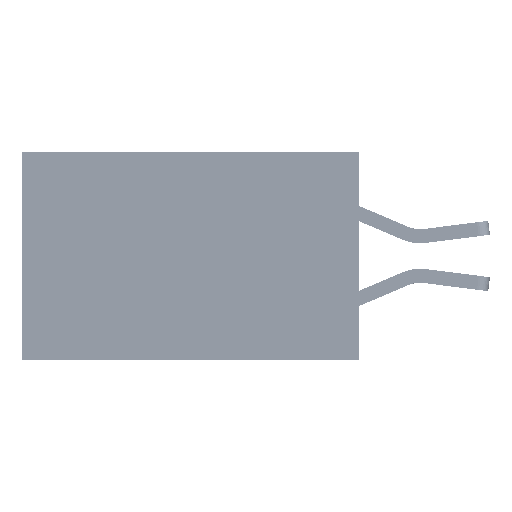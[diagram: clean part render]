
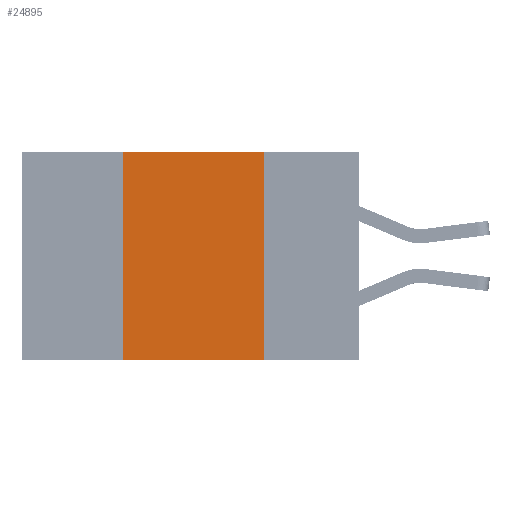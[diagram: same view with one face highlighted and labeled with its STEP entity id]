
A CAD part, left-side view. The second image highlights one B-rep face of the part: STEP entity #24895.
In plain terms, the highlighted planar face has unit normal (-1, 0, 0).
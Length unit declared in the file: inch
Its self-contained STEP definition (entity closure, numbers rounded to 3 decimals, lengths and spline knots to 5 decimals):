
#4456 = LINE ( 'NONE', #37391, #8696 ) ;
#4467 = CARTESIAN_POINT ( 'NONE',  ( 0., 0.42, 0. ) ) ;
#5100 = EDGE_CURVE ( 'NONE', #24556, #27196, #4456, .T. ) ;
#7430 = VERTEX_POINT ( 'NONE', #36859 ) ;
#7433 = EDGE_CURVE ( 'NONE', #27196, #11251, #16184, .T. ) ;
#8696 = VECTOR ( 'NONE', #29924, 39.37008 ) ;
#11251 = VERTEX_POINT ( 'NONE', #30616 ) ;
#11850 = CARTESIAN_POINT ( 'NONE',  ( 0., 0.42, 0. ) ) ;
#12069 = DIRECTION ( 'NONE',  ( 0., 0., -1. ) ) ;
#12838 = CARTESIAN_POINT ( 'NONE',  ( 0., 0.6, -0.37 ) ) ;
#15282 = PLANE ( 'NONE',  #31566 ) ;
#16184 = LINE ( 'NONE', #26851, #38500 ) ;
#18351 = EDGE_CURVE ( 'NONE', #7430, #11251, #19217, .T. ) ;
#18672 = DIRECTION ( 'NONE',  ( 1., 0., 0. ) ) ;
#18903 = CARTESIAN_POINT ( 'NONE',  ( 0., 0.6, 0. ) ) ;
#19217 = LINE ( 'NONE', #12838, #21851 ) ;
#21851 = VECTOR ( 'NONE', #36947, 39.37008 ) ;
#24014 = EDGE_LOOP ( 'NONE', ( #31407, #38094, #44528, #39488 ) ) ;
#24556 = VERTEX_POINT ( 'NONE', #4467 ) ;
#24895 = ADVANCED_FACE ( 'NONE', ( #25041 ), #15282, .F. ) ;
#25041 = FACE_OUTER_BOUND ( 'NONE', #24014, .T. ) ;
#26851 = CARTESIAN_POINT ( 'NONE',  ( 0., 0.17, 0. ) ) ;
#27196 = VERTEX_POINT ( 'NONE', #36301 ) ;
#29924 = DIRECTION ( 'NONE',  ( 0., -1., 0. ) ) ;
#30616 = CARTESIAN_POINT ( 'NONE',  ( 0., 0.17, -0.37 ) ) ;
#31058 = EDGE_CURVE ( 'NONE', #7430, #24556, #38883, .T. ) ;
#31407 = ORIENTED_EDGE ( 'NONE', *, *, #7433, .F. ) ;
#31566 = AXIS2_PLACEMENT_3D ( 'NONE', #18903, #18672, #12069 ) ;
#33224 = DIRECTION ( 'NONE',  ( 0., 0., -1. ) ) ;
#34485 = VECTOR ( 'NONE', #38669, 39.37008 ) ;
#36301 = CARTESIAN_POINT ( 'NONE',  ( 0., 0.17, 0. ) ) ;
#36859 = CARTESIAN_POINT ( 'NONE',  ( 0., 0.42, -0.37 ) ) ;
#36947 = DIRECTION ( 'NONE',  ( 0., -1., 0. ) ) ;
#37391 = CARTESIAN_POINT ( 'NONE',  ( 0., 0.6, 0. ) ) ;
#38094 = ORIENTED_EDGE ( 'NONE', *, *, #5100, .F. ) ;
#38500 = VECTOR ( 'NONE', #33224, 39.37008 ) ;
#38669 = DIRECTION ( 'NONE',  ( 0., 0., 1. ) ) ;
#38883 = LINE ( 'NONE', #11850, #34485 ) ;
#39488 = ORIENTED_EDGE ( 'NONE', *, *, #18351, .T. ) ;
#44528 = ORIENTED_EDGE ( 'NONE', *, *, #31058, .F. ) ;
